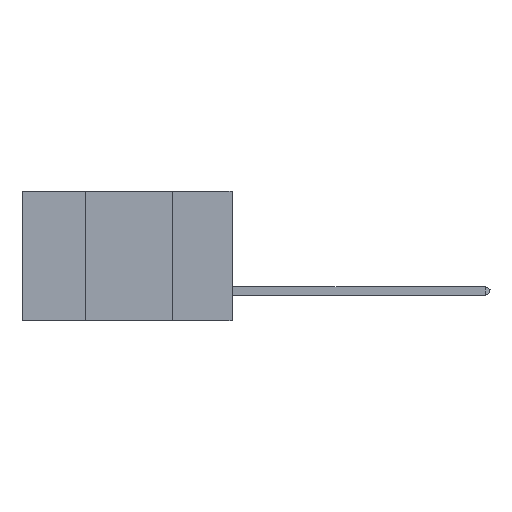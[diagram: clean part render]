
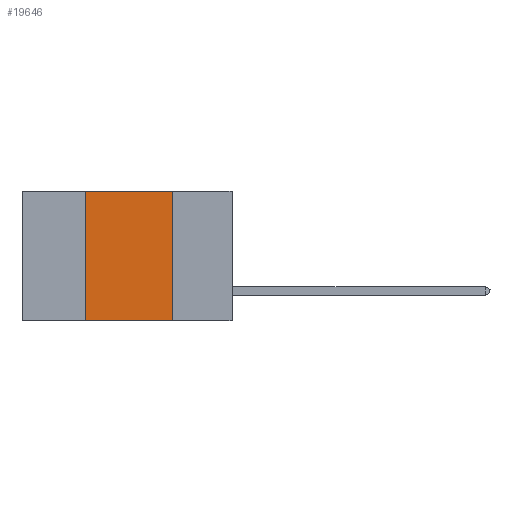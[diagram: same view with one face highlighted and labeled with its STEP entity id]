
A CAD part, left-side view. The second image highlights one B-rep face of the part: STEP entity #19646.
In plain terms, the highlighted planar face has unit normal (-1, 0, 0).
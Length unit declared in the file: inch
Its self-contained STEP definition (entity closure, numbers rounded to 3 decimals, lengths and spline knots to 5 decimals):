
#7 = CARTESIAN_POINT ( 'NONE',  ( 0., 0.42, -0.37 ) ) ;
#696 = VERTEX_POINT ( 'NONE', #19633 ) ;
#1028 = VERTEX_POINT ( 'NONE', #7969 ) ;
#4252 = CARTESIAN_POINT ( 'NONE',  ( 0., 0.6, -0.37 ) ) ;
#4504 = ORIENTED_EDGE ( 'NONE', *, *, #7840, .F. ) ;
#4774 = VECTOR ( 'NONE', #29641, 39.37008 ) ;
#7840 = EDGE_CURVE ( 'NONE', #22894, #696, #14582, .T. ) ;
#7969 = CARTESIAN_POINT ( 'NONE',  ( 0., 0.17, 0. ) ) ;
#9699 = CARTESIAN_POINT ( 'NONE',  ( 0., 0.6, 0. ) ) ;
#9915 = EDGE_CURVE ( 'NONE', #22894, #18286, #12344, .T. ) ;
#11896 = DIRECTION ( 'NONE',  ( 0., 0., -1. ) ) ;
#12344 = LINE ( 'NONE', #4252, #4774 ) ;
#14108 = PLANE ( 'NONE',  #15685 ) ;
#14582 = LINE ( 'NONE', #28931, #19594 ) ;
#14830 = VECTOR ( 'NONE', #21351, 39.37008 ) ;
#15685 = AXIS2_PLACEMENT_3D ( 'NONE', #21006, #25420, #11896 ) ;
#16121 = EDGE_LOOP ( 'NONE', ( #23684, #18397, #4504, #22330 ) ) ;
#18286 = VERTEX_POINT ( 'NONE', #29547 ) ;
#18397 = ORIENTED_EDGE ( 'NONE', *, *, #22461, .F. ) ;
#19594 = VECTOR ( 'NONE', #22403, 39.37008 ) ;
#19633 = CARTESIAN_POINT ( 'NONE',  ( 0., 0.42, 0. ) ) ;
#19646 = ADVANCED_FACE ( 'NONE', ( #24615 ), #14108, .F. ) ;
#21006 = CARTESIAN_POINT ( 'NONE',  ( 0., 0.6, 0. ) ) ;
#21351 = DIRECTION ( 'NONE',  ( 0., 0., -1. ) ) ;
#22330 = ORIENTED_EDGE ( 'NONE', *, *, #9915, .T. ) ;
#22403 = DIRECTION ( 'NONE',  ( 0., 0., 1. ) ) ;
#22461 = EDGE_CURVE ( 'NONE', #696, #1028, #23383, .T. ) ;
#22894 = VERTEX_POINT ( 'NONE', #7 ) ;
#23383 = LINE ( 'NONE', #9699, #28781 ) ;
#23684 = ORIENTED_EDGE ( 'NONE', *, *, #28269, .F. ) ;
#23761 = LINE ( 'NONE', #28050, #14830 ) ;
#24615 = FACE_OUTER_BOUND ( 'NONE', #16121, .T. ) ;
#25420 = DIRECTION ( 'NONE',  ( 1., 0., 0. ) ) ;
#27992 = DIRECTION ( 'NONE',  ( 0., -1., 0. ) ) ;
#28050 = CARTESIAN_POINT ( 'NONE',  ( 0., 0.17, 0. ) ) ;
#28269 = EDGE_CURVE ( 'NONE', #1028, #18286, #23761, .T. ) ;
#28781 = VECTOR ( 'NONE', #27992, 39.37008 ) ;
#28931 = CARTESIAN_POINT ( 'NONE',  ( 0., 0.42, 0. ) ) ;
#29547 = CARTESIAN_POINT ( 'NONE',  ( 0., 0.17, -0.37 ) ) ;
#29641 = DIRECTION ( 'NONE',  ( 0., -1., 0. ) ) ;
